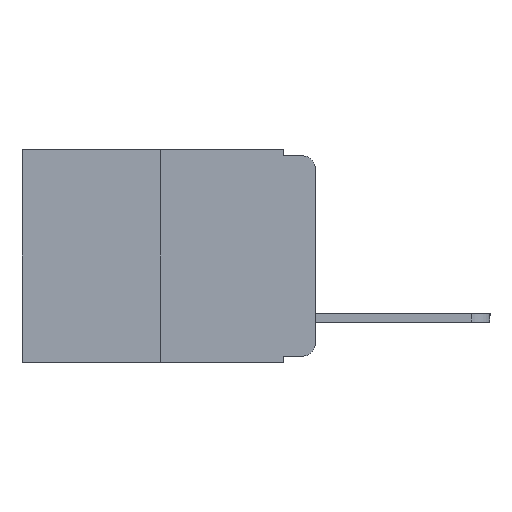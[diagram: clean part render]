
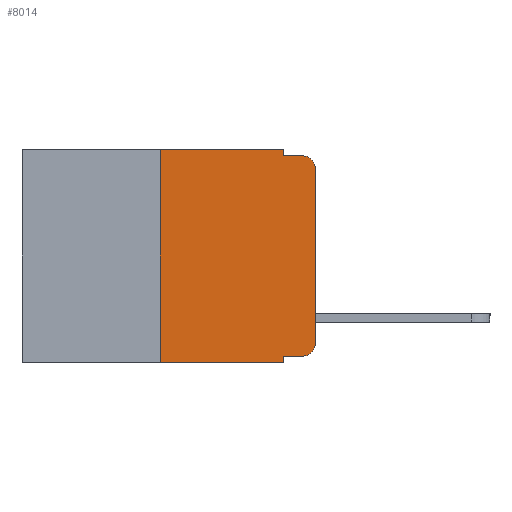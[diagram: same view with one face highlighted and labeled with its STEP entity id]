
A CAD part, left-side view. The second image highlights one B-rep face of the part: STEP entity #8014.
In plain terms, the highlighted planar face has unit normal (-1, 0, 0).
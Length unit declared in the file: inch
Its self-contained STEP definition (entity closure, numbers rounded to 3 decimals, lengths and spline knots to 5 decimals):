
#101 = EDGE_CURVE ( 'NONE', #11650, #12278, #5939, .T. ) ;
#107 = AXIS2_PLACEMENT_3D ( 'NONE', #4884, #16822, #6695 ) ;
#639 = LINE ( 'NONE', #1098, #14861 ) ;
#894 = VECTOR ( 'NONE', #14970, 39.37008 ) ;
#917 = VERTEX_POINT ( 'NONE', #985 ) ;
#985 = CARTESIAN_POINT ( 'NONE',  ( 0., 0., -0.313 ) ) ;
#1098 = CARTESIAN_POINT ( 'NONE',  ( 0., 0.051, -0.01 ) ) ;
#1121 = EDGE_CURVE ( 'NONE', #15925, #4803, #10549, .T. ) ;
#1957 = DIRECTION ( 'NONE',  ( 0., -1., 0. ) ) ;
#2028 = CARTESIAN_POINT ( 'NONE',  ( 0., 0.02, -0.333 ) ) ;
#2030 = EDGE_CURVE ( 'NONE', #917, #21884, #16381, .T. ) ;
#2085 = EDGE_CURVE ( 'NONE', #21884, #6570, #10475, .T. ) ;
#2090 = EDGE_CURVE ( 'NONE', #12240, #6570, #639, .T. ) ;
#2121 = EDGE_CURVE ( 'NONE', #12278, #12240, #13805, .T. ) ;
#2163 = EDGE_CURVE ( 'NONE', #15925, #11650, #4583, .T. ) ;
#2283 = EDGE_CURVE ( 'NONE', #9627, #4803, #15616, .T. ) ;
#2371 = EDGE_CURVE ( 'NONE', #9627, #18893, #12264, .T. ) ;
#2375 = EDGE_CURVE ( 'NONE', #18893, #917, #10202, .T. ) ;
#2436 = ORIENTED_EDGE ( 'NONE', *, *, #2121, .F. ) ;
#3347 = ORIENTED_EDGE ( 'NONE', *, *, #2030, .T. ) ;
#3652 = ORIENTED_EDGE ( 'NONE', *, *, #101, .F. ) ;
#3877 = CARTESIAN_POINT ( 'NONE',  ( 0., 0.051, -0.333 ) ) ;
#3952 = DIRECTION ( 'NONE',  ( -1., 0., 0. ) ) ;
#4583 = LINE ( 'NONE', #15440, #21298 ) ;
#4730 = DIRECTION ( 'NONE',  ( 0., 0., -1. ) ) ;
#4803 = VERTEX_POINT ( 'NONE', #6466 ) ;
#4884 = CARTESIAN_POINT ( 'NONE',  ( 0., 0.02, -0.03 ) ) ;
#5145 = VECTOR ( 'NONE', #21642, 39.37008 ) ;
#5423 = CARTESIAN_POINT ( 'NONE',  ( 0., 0.051, 0. ) ) ;
#5670 = ORIENTED_EDGE ( 'NONE', *, *, #2375, .T. ) ;
#5939 = LINE ( 'NONE', #14989, #894 ) ;
#6466 = CARTESIAN_POINT ( 'NONE',  ( 0., 0.051, -0.343 ) ) ;
#6570 = VERTEX_POINT ( 'NONE', #16647 ) ;
#6589 = AXIS2_PLACEMENT_3D ( 'NONE', #19799, #15081, #4730 ) ;
#6695 = DIRECTION ( 'NONE',  ( 0., 0., -1. ) ) ;
#6787 = ORIENTED_EDGE ( 'NONE', *, *, #2090, .F. ) ;
#8014 = ADVANCED_FACE ( 'NONE', ( #8861 ), #13404, .F. ) ;
#8183 = ORIENTED_EDGE ( 'NONE', *, *, #2085, .T. ) ;
#8861 = FACE_OUTER_BOUND ( 'NONE', #12959, .T. ) ;
#9255 = CARTESIAN_POINT ( 'NONE',  ( 0., 0.051, -0.01 ) ) ;
#9627 = VERTEX_POINT ( 'NONE', #16319 ) ;
#9657 = AXIS2_PLACEMENT_3D ( 'NONE', #14386, #3952, #16016 ) ;
#10017 = VECTOR ( 'NONE', #13367, 39.37008 ) ;
#10202 = CIRCLE ( 'NONE', #9657, 0.02 ) ;
#10475 = CIRCLE ( 'NONE', #107, 0.02 ) ;
#10549 = LINE ( 'NONE', #21344, #10017 ) ;
#11246 = VECTOR ( 'NONE', #18890, 39.37008 ) ;
#11650 = VERTEX_POINT ( 'NONE', #21027 ) ;
#11709 = ORIENTED_EDGE ( 'NONE', *, *, #1121, .T. ) ;
#12240 = VERTEX_POINT ( 'NONE', #9255 ) ;
#12264 = LINE ( 'NONE', #3877, #17854 ) ;
#12278 = VERTEX_POINT ( 'NONE', #20684 ) ;
#12959 = EDGE_LOOP ( 'NONE', ( #3347, #8183, #6787, #2436, #3652, #14571, #11709, #16100, #17102, #5670 ) ) ;
#13367 = DIRECTION ( 'NONE',  ( 0., -1., 0. ) ) ;
#13404 = PLANE ( 'NONE',  #6589 ) ;
#13731 = DIRECTION ( 'NONE',  ( 0., 0., 1. ) ) ;
#13805 = LINE ( 'NONE', #16986, #5145 ) ;
#14386 = CARTESIAN_POINT ( 'NONE',  ( 0., 0.02, -0.313 ) ) ;
#14571 = ORIENTED_EDGE ( 'NONE', *, *, #2163, .F. ) ;
#14861 = VECTOR ( 'NONE', #19991, 39.37008 ) ;
#14970 = DIRECTION ( 'NONE',  ( 0., -1., 0. ) ) ;
#14989 = CARTESIAN_POINT ( 'NONE',  ( 0., 0.473, 0. ) ) ;
#15081 = DIRECTION ( 'NONE',  ( 1., 0., 0. ) ) ;
#15184 = CARTESIAN_POINT ( 'NONE',  ( 0., 0., -0.03 ) ) ;
#15440 = CARTESIAN_POINT ( 'NONE',  ( 0., 0.25, 0. ) ) ;
#15472 = CARTESIAN_POINT ( 'NONE',  ( 0., 0.25, -0.343 ) ) ;
#15616 = LINE ( 'NONE', #5423, #11246 ) ;
#15925 = VERTEX_POINT ( 'NONE', #15472 ) ;
#16016 = DIRECTION ( 'NONE',  ( 0., 0., -1. ) ) ;
#16100 = ORIENTED_EDGE ( 'NONE', *, *, #2283, .F. ) ;
#16319 = CARTESIAN_POINT ( 'NONE',  ( 0., 0.051, -0.333 ) ) ;
#16381 = LINE ( 'NONE', #18225, #20102 ) ;
#16647 = CARTESIAN_POINT ( 'NONE',  ( 0., 0.02, -0.01 ) ) ;
#16822 = DIRECTION ( 'NONE',  ( -1., 0., 0. ) ) ;
#16986 = CARTESIAN_POINT ( 'NONE',  ( 0., 0.051, 0. ) ) ;
#17102 = ORIENTED_EDGE ( 'NONE', *, *, #2371, .T. ) ;
#17854 = VECTOR ( 'NONE', #1957, 39.37008 ) ;
#18225 = CARTESIAN_POINT ( 'NONE',  ( 0., 0., 0. ) ) ;
#18890 = DIRECTION ( 'NONE',  ( 0., 0., -1. ) ) ;
#18893 = VERTEX_POINT ( 'NONE', #2028 ) ;
#19783 = DIRECTION ( 'NONE',  ( 0., 0., 1. ) ) ;
#19799 = CARTESIAN_POINT ( 'NONE',  ( 0., 0.473, 0. ) ) ;
#19991 = DIRECTION ( 'NONE',  ( 0., -1., 0. ) ) ;
#20102 = VECTOR ( 'NONE', #19783, 39.37008 ) ;
#20684 = CARTESIAN_POINT ( 'NONE',  ( 0., 0.051, 0. ) ) ;
#21027 = CARTESIAN_POINT ( 'NONE',  ( 0., 0.25, 0. ) ) ;
#21298 = VECTOR ( 'NONE', #13731, 39.37008 ) ;
#21344 = CARTESIAN_POINT ( 'NONE',  ( 0., 0.473, -0.343 ) ) ;
#21642 = DIRECTION ( 'NONE',  ( 0., 0., -1. ) ) ;
#21884 = VERTEX_POINT ( 'NONE', #15184 ) ;
